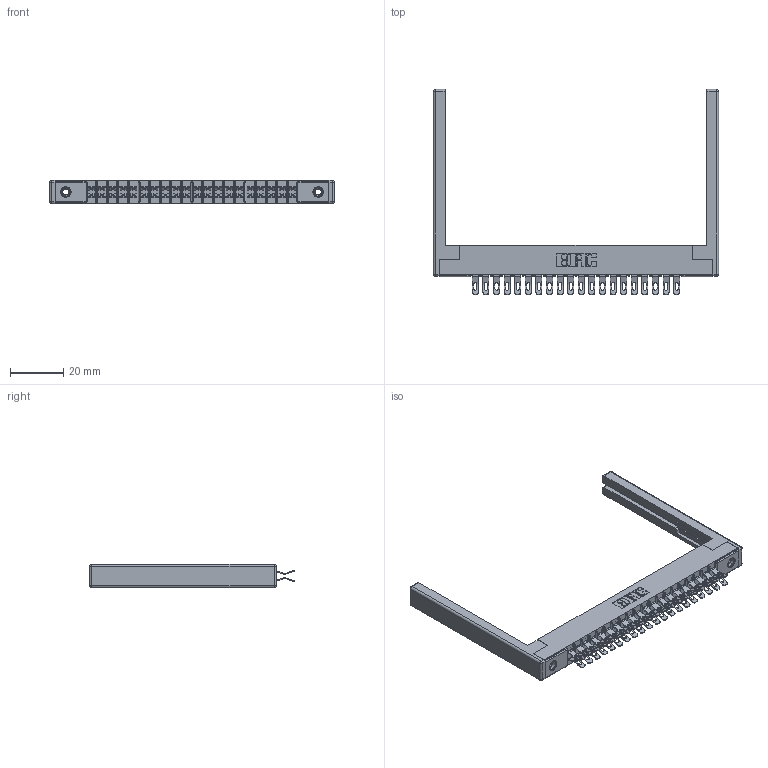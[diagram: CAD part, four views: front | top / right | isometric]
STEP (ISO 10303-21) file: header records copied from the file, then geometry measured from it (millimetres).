
FILE_DESCRIPTION (( 'STEP AP203' ), '1' );
FILE_NAME ('305-040-555-568.STEP', '2019-09-09T19:09:09', ( '' ), ( '' ), 'SwSTEP 2.0', 'SolidWorks 2016', '' );
FILE_SCHEMA (( 'CONFIG_CONTROL_DESIGN' ));
Length unit declared in the file: inch
Products named in the file (5): 305 Part_.156 Dia; 305-040-555-568; 345-250-001_345-250-001-102; 307-220-068; 305-290-001_555
Assembly tree (45 placements, depth 2):
  305-040-555-568
    305 Part_.156 Dia
    305-290-001_555  x40
    345-250-001_345-250-001-102  x2
    307-220-068  x2
Bounding box: 106.68 x 76.71 x 8.71 mm (x, y, z)
Volume: 11104.5 mm3; surface area: 17552.3 mm2
Topology: 45 solids, 45 shells, 2910 faces, 8606 edges, 5608 vertices
Faces by surface type: plane 1436, cylinder 1370, sphere 88, cone 12, torus 4
Entity records: 27716 total; most frequent: CARTESIAN_POINT 4577, ORIENTED_EDGE 4522, DIRECTION 4459, EDGE_CURVE 2261, LINE 1775, VECTOR 1775, VERTEX_POINT 1444, AXIS2_PLACEMENT_3D 1342
